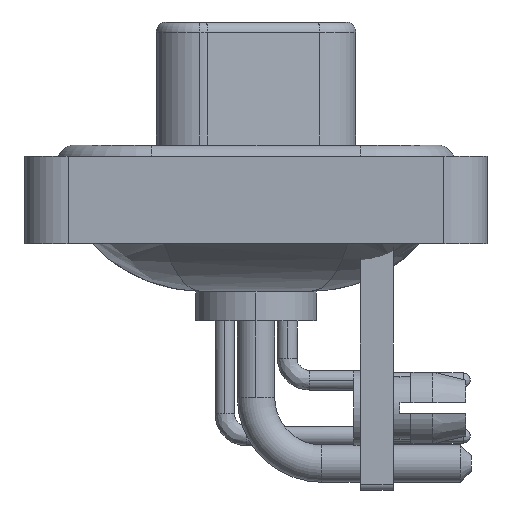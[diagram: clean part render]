
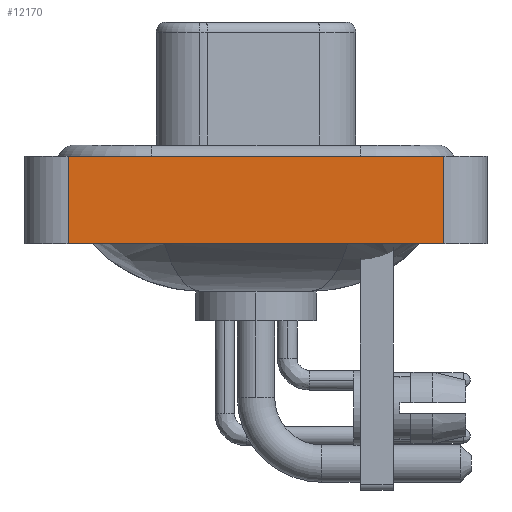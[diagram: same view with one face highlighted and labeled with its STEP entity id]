
A CAD part, left-side view. The second image highlights one B-rep face of the part: STEP entity #12170.
In plain terms, the highlighted planar face has unit normal (-1, 0, 0).
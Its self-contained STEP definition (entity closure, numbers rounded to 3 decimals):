
#166 = CARTESIAN_POINT ( 'NONE',  ( -7.35, -8.55, -3.6 ) ) ;
#712 = CARTESIAN_POINT ( 'NONE',  ( -7.35, -8.55, 0.4 ) ) ;
#858 = LINE ( 'NONE', #712, #17481 ) ;
#1227 = DIRECTION ( 'NONE',  ( 0., 0., 1. ) ) ;
#1649 = CARTESIAN_POINT ( 'NONE',  ( -7.35, 8.55, 0.4 ) ) ;
#3519 = DIRECTION ( 'NONE',  ( 0., -1., 0. ) ) ;
#4197 = AXIS2_PLACEMENT_3D ( 'NONE', #5891, #12832, #25920 ) ;
#5398 = EDGE_CURVE ( 'NONE', #26906, #16967, #12224, .T. ) ;
#5526 = VERTEX_POINT ( 'NONE', #1649 ) ;
#5891 = CARTESIAN_POINT ( 'NONE',  ( -7.35, -8.55, -3.6 ) ) ;
#6860 = LINE ( 'NONE', #15520, #21914 ) ;
#7623 = CARTESIAN_POINT ( 'NONE',  ( -7.35, -8.55, 0.4 ) ) ;
#9172 = DIRECTION ( 'NONE',  ( 0., 0., 1. ) ) ;
#9719 = EDGE_CURVE ( 'NONE', #5526, #16967, #858, .T. ) ;
#9963 = DIRECTION ( 'NONE',  ( 0., -1., 0. ) ) ;
#10357 = VECTOR ( 'NONE', #3519, 1000. ) ;
#11234 = ORIENTED_EDGE ( 'NONE', *, *, #5398, .T. ) ;
#12069 = CARTESIAN_POINT ( 'NONE',  ( -7.35, -8.55, -3.6 ) ) ;
#12170 = ADVANCED_FACE ( 'NONE', ( #12406 ), #23203, .T. ) ;
#12224 = LINE ( 'NONE', #14100, #24245 ) ;
#12406 = FACE_OUTER_BOUND ( 'NONE', #13149, .T. ) ;
#12832 = DIRECTION ( 'NONE',  ( -1., 0., 0. ) ) ;
#12853 = CARTESIAN_POINT ( 'NONE',  ( -7.35, 8.55, -3.6 ) ) ;
#13149 = EDGE_LOOP ( 'NONE', ( #11234, #22729, #14930, #21293 ) ) ;
#14100 = CARTESIAN_POINT ( 'NONE',  ( -7.35, -8.55, -3.6 ) ) ;
#14930 = ORIENTED_EDGE ( 'NONE', *, *, #18975, .F. ) ;
#15520 = CARTESIAN_POINT ( 'NONE',  ( -7.35, 8.55, -3.6 ) ) ;
#16967 = VERTEX_POINT ( 'NONE', #7623 ) ;
#17481 = VECTOR ( 'NONE', #9963, 1000. ) ;
#18975 = EDGE_CURVE ( 'NONE', #27105, #5526, #6860, .T. ) ;
#20996 = LINE ( 'NONE', #12069, #10357 ) ;
#21293 = ORIENTED_EDGE ( 'NONE', *, *, #28407, .T. ) ;
#21914 = VECTOR ( 'NONE', #9172, 1000. ) ;
#22729 = ORIENTED_EDGE ( 'NONE', *, *, #9719, .F. ) ;
#23203 = PLANE ( 'NONE',  #4197 ) ;
#24245 = VECTOR ( 'NONE', #1227, 1000. ) ;
#25920 = DIRECTION ( 'NONE',  ( 0., 0., 1. ) ) ;
#26906 = VERTEX_POINT ( 'NONE', #166 ) ;
#27105 = VERTEX_POINT ( 'NONE', #12853 ) ;
#28407 = EDGE_CURVE ( 'NONE', #27105, #26906, #20996, .T. ) ;
